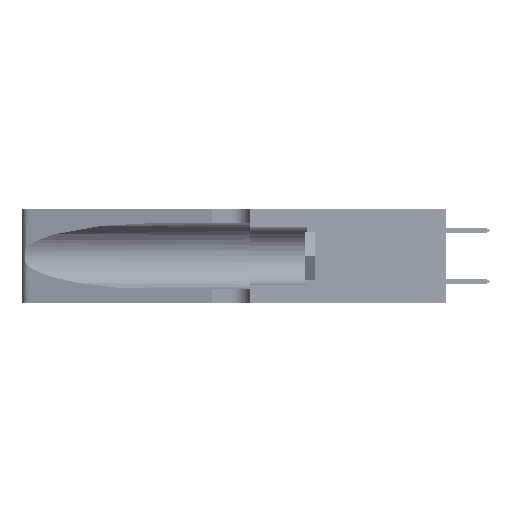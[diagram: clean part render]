
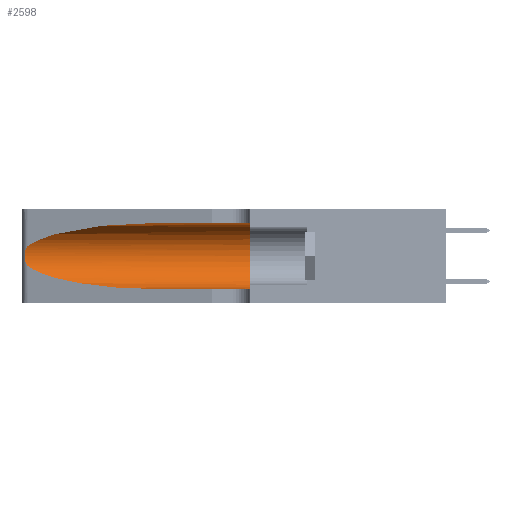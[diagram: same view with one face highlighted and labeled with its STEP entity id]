
A CAD part, left-side view. The second image highlights one B-rep face of the part: STEP entity #2598.
In plain terms, the highlighted cylindrical face has radius 3.308 mm (diameter 6.617 mm), a partial arc.
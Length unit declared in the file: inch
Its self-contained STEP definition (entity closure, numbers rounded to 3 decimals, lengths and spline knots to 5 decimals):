
#420 = DIRECTION ( 'NONE',  ( 0., -1., 0. ) ) ;
#1807 = CARTESIAN_POINT ( 'NONE',  ( 0.25555, 1.22994, 0.2215 ) ) ;
#1969 = CARTESIAN_POINT ( 'NONE',  ( 0.26075, 1.23896, 0.19203 ) ) ;
#2156 = CARTESIAN_POINT ( 'NONE',  ( 0.25487, 1.22718, 0.14631 ) ) ;
#2598 = ADVANCED_FACE ( 'NONE', ( #33898 ), #22979, .F. ) ;
#4034 = ORIENTED_EDGE ( 'NONE', *, *, #45461, .T. ) ;
#4046 = CARTESIAN_POINT ( 'NONE',  ( 0.1305, 0.72297, 0.05475 ) ) ;
#4156 = CARTESIAN_POINT ( 'NONE',  ( 0.1305, 1.61858, 0.31525 ) ) ;
#4591 = CIRCLE ( 'NONE', #19201, 0.13025 ) ;
#5730 = CARTESIAN_POINT ( 'NONE',  ( 0.26017, 1.23833, 0.17102 ) ) ;
#6008 = VERTEX_POINT ( 'NONE', #16225 ) ;
#6962 = CARTESIAN_POINT ( 'NONE',  ( 0.1305, 0.35, 0.185 ) ) ;
#7139 = B_SPLINE_CURVE_WITH_KNOTS ( 'NONE', 3,
 ( #20290, #1807, #42442, #20432, #46117, #24162, #1969, #27812, #5730, #31532, #9435, #35249, #13153, #38911 ),
 .UNSPECIFIED., .F., .F.,
 ( 4, 2, 2, 2, 2, 2, 4 ),
 ( 0., 0.00027, 0.00053, 0.00107, 0.0016, 0.00187, 0.00214 ),
 .UNSPECIFIED. ) ;
#8929 = CARTESIAN_POINT ( 'NONE',  ( 0.25487, 1.22718, 0.22369 ) ) ;
#9284 = ORIENTED_EDGE ( 'NONE', *, *, #33061, .T. ) ;
#9435 = CARTESIAN_POINT ( 'NONE',  ( 0.25789, 1.23486, 0.15765 ) ) ;
#9932 = ORIENTED_EDGE ( 'NONE', *, *, #17995, .F. ) ;
#10670 = DIRECTION ( 'NONE',  ( 0., 0., 1. ) ) ;
#12160 =( BOUNDED_CURVE ( )  B_SPLINE_CURVE ( 3, ( #16193, #38267, #31040, #8929 ),
 .UNSPECIFIED., .F., .F. ) 
 B_SPLINE_CURVE_WITH_KNOTS ( ( 4, 4 ),
 ( 1.5708, 2.84003 ),
 .UNSPECIFIED. ) 
 CURVE ( )  GEOMETRIC_REPRESENTATION_ITEM ( )  RATIONAL_B_SPLINE_CURVE ( ( 1., 0.87, 0.87, 1. ) ) 
 REPRESENTATION_ITEM ( '' )  );
#13153 = CARTESIAN_POINT ( 'NONE',  ( 0.25555, 1.22993, 0.14849 ) ) ;
#14303 = AXIS2_PLACEMENT_3D ( 'NONE', #19122, #41149, #33775 ) ;
#15775 = CARTESIAN_POINT ( 'NONE',  ( 0.1305, 0.35, 0.05475 ) ) ;
#16193 = CARTESIAN_POINT ( 'NONE',  ( 0.1305, 0.72297, 0.31525 ) ) ;
#16225 = CARTESIAN_POINT ( 'NONE',  ( 0.1305, 0.35, 0.31525 ) ) ;
#16326 = CARTESIAN_POINT ( 'NONE',  ( 0.18966, 0.96281, 0.05475 ) ) ;
#17442 = ORIENTED_EDGE ( 'NONE', *, *, #35770, .F. ) ;
#17995 = EDGE_CURVE ( 'NONE', #35053, #6008, #46662, .T. ) ;
#19122 = CARTESIAN_POINT ( 'NONE',  ( 0.1305, 1.61858, 0.185 ) ) ;
#19201 = AXIS2_PLACEMENT_3D ( 'NONE', #6962, #32772, #10670 ) ;
#20290 = CARTESIAN_POINT ( 'NONE',  ( 0.25487, 1.22718, 0.22369 ) ) ;
#20432 = CARTESIAN_POINT ( 'NONE',  ( 0.25787, 1.23484, 0.2124 ) ) ;
#20586 = VECTOR ( 'NONE', #28332, 39.37008 ) ;
#22979 = CYLINDRICAL_SURFACE ( 'NONE', #14303, 0.13025 ) ;
#24162 = CARTESIAN_POINT ( 'NONE',  ( 0.26018, 1.23835, 0.19895 ) ) ;
#24347 =( BOUNDED_CURVE ( )  B_SPLINE_CURVE ( 3, ( #34738, #38408, #16326, #42081 ),
 .UNSPECIFIED., .F., .T. ) 
 B_SPLINE_CURVE_WITH_KNOTS ( ( 4, 4 ),
 ( 3.44316, 4.71239 ),
 .UNSPECIFIED. ) 
 CURVE ( )  GEOMETRIC_REPRESENTATION_ITEM ( )  RATIONAL_B_SPLINE_CURVE ( ( 1., 0.87, 0.87, 1. ) ) 
 REPRESENTATION_ITEM ( '' )  );
#25186 = VERTEX_POINT ( 'NONE', #2156 ) ;
#25780 = VERTEX_POINT ( 'NONE', #38413 ) ;
#27134 = VECTOR ( 'NONE', #420, 39.37008 ) ;
#27812 = CARTESIAN_POINT ( 'NONE',  ( 0.26075, 1.23896, 0.178 ) ) ;
#28332 = DIRECTION ( 'NONE',  ( 0., -1., 0. ) ) ;
#31040 = CARTESIAN_POINT ( 'NONE',  ( 0.2373, 1.15595, 0.28018 ) ) ;
#31532 = CARTESIAN_POINT ( 'NONE',  ( 0.25856, 1.23593, 0.16098 ) ) ;
#32772 = DIRECTION ( 'NONE',  ( 0., 1., 0. ) ) ;
#33061 = EDGE_CURVE ( 'NONE', #25186, #43885, #24347, .T. ) ;
#33775 = DIRECTION ( 'NONE',  ( 0., 0., -1. ) ) ;
#33898 = FACE_OUTER_BOUND ( 'NONE', #39013, .T. ) ;
#34665 = ORIENTED_EDGE ( 'NONE', *, *, #38438, .T. ) ;
#34738 = CARTESIAN_POINT ( 'NONE',  ( 0.25487, 1.22718, 0.14631 ) ) ;
#35053 = VERTEX_POINT ( 'NONE', #42589 ) ;
#35249 = CARTESIAN_POINT ( 'NONE',  ( 0.25639, 1.23186, 0.15144 ) ) ;
#35770 = EDGE_CURVE ( 'NONE', #6008, #39620, #4591, .T. ) ;
#38267 = CARTESIAN_POINT ( 'NONE',  ( 0.18966, 0.96281, 0.31525 ) ) ;
#38408 = CARTESIAN_POINT ( 'NONE',  ( 0.2373, 1.15595, 0.08982 ) ) ;
#38413 = CARTESIAN_POINT ( 'NONE',  ( 0.25487, 1.22718, 0.22369 ) ) ;
#38438 = EDGE_CURVE ( 'NONE', #25780, #25186, #7139, .T. ) ;
#38911 = CARTESIAN_POINT ( 'NONE',  ( 0.25487, 1.22718, 0.14631 ) ) ;
#39013 = EDGE_LOOP ( 'NONE', ( #4034, #34665, #9284, #41582, #17442, #9932 ) ) ;
#39620 = VERTEX_POINT ( 'NONE', #15775 ) ;
#40147 = LINE ( 'NONE', #42963, #20586 ) ;
#41149 = DIRECTION ( 'NONE',  ( 0., -1., 0. ) ) ;
#41582 = ORIENTED_EDGE ( 'NONE', *, *, #42701, .T. ) ;
#42081 = CARTESIAN_POINT ( 'NONE',  ( 0.1305, 0.72297, 0.05475 ) ) ;
#42442 = CARTESIAN_POINT ( 'NONE',  ( 0.25639, 1.23184, 0.21858 ) ) ;
#42589 = CARTESIAN_POINT ( 'NONE',  ( 0.1305, 0.72297, 0.31525 ) ) ;
#42701 = EDGE_CURVE ( 'NONE', #43885, #39620, #40147, .T. ) ;
#42963 = CARTESIAN_POINT ( 'NONE',  ( 0.1305, 1.61858, 0.05475 ) ) ;
#43885 = VERTEX_POINT ( 'NONE', #4046 ) ;
#45461 = EDGE_CURVE ( 'NONE', #35053, #25780, #12160, .T. ) ;
#46117 = CARTESIAN_POINT ( 'NONE',  ( 0.25854, 1.2359, 0.20912 ) ) ;
#46662 = LINE ( 'NONE', #4156, #27134 ) ;
